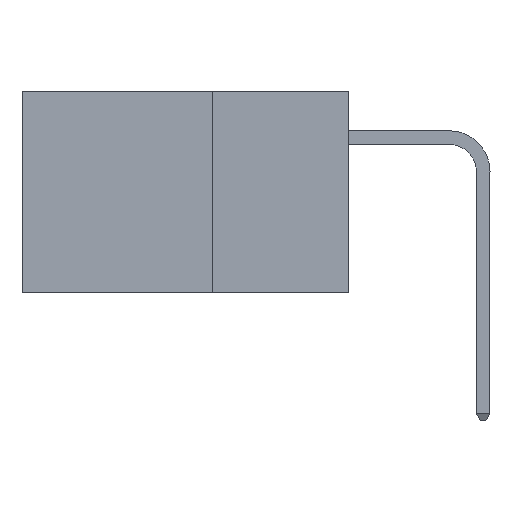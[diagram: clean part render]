
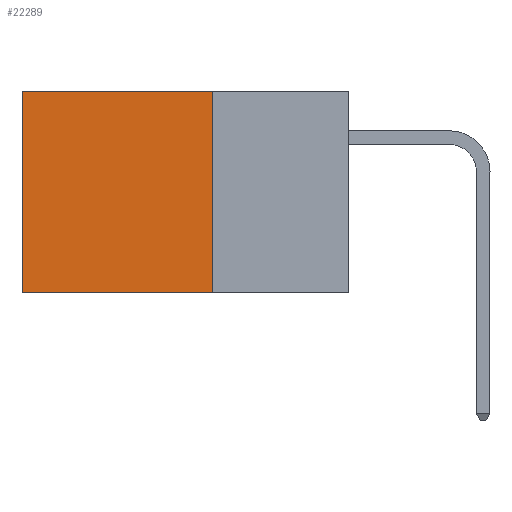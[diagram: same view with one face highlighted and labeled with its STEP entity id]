
A CAD part, left-side view. The second image highlights one B-rep face of the part: STEP entity #22289.
In plain terms, the highlighted planar face has unit normal (-1, 0, 0).
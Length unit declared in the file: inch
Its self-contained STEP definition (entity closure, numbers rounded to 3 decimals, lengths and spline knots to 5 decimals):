
#1693 = ORIENTED_EDGE ( 'NONE', *, *, #2872, .T. ) ;
#2872 = EDGE_CURVE ( 'NONE', #6135, #3264, #35801, .T. ) ;
#3264 = VERTEX_POINT ( 'NONE', #6085 ) ;
#6085 = CARTESIAN_POINT ( 'NONE',  ( 0.2875, 0.6, -0.37 ) ) ;
#6135 = VERTEX_POINT ( 'NONE', #34366 ) ;
#6524 = CARTESIAN_POINT ( 'NONE',  ( 0.2875, 0.25, -0.37 ) ) ;
#7345 = EDGE_CURVE ( 'NONE', #34507, #6135, #17134, .T. ) ;
#7349 = EDGE_CURVE ( 'NONE', #34507, #25520, #25265, .T. ) ;
#9514 = VECTOR ( 'NONE', #26277, 39.37008 ) ;
#9558 = CARTESIAN_POINT ( 'NONE',  ( 0.2875, 0.25, 0. ) ) ;
#9845 = DIRECTION ( 'NONE',  ( 1., 0., 0. ) ) ;
#12201 = VECTOR ( 'NONE', #18592, 39.37008 ) ;
#14779 = EDGE_LOOP ( 'NONE', ( #1693, #34271, #35120, #15845 ) ) ;
#15296 = DIRECTION ( 'NONE',  ( 0., 1., 0. ) ) ;
#15591 = AXIS2_PLACEMENT_3D ( 'NONE', #26546, #9845, #29298 ) ;
#15845 = ORIENTED_EDGE ( 'NONE', *, *, #7345, .T. ) ;
#17134 = LINE ( 'NONE', #31594, #9514 ) ;
#18055 = CARTESIAN_POINT ( 'NONE',  ( 0.2875, 0.25, -0.37 ) ) ;
#18592 = DIRECTION ( 'NONE',  ( 0., 0., -1. ) ) ;
#19849 = CARTESIAN_POINT ( 'NONE',  ( 0.2875, 0.25, 0. ) ) ;
#20253 = EDGE_CURVE ( 'NONE', #25520, #3264, #30960, .T. ) ;
#22289 = ADVANCED_FACE ( 'NONE', ( #27917 ), #34545, .F. ) ;
#23713 = VECTOR ( 'NONE', #15296, 39.37008 ) ;
#25265 = LINE ( 'NONE', #9558, #30795 ) ;
#25520 = VERTEX_POINT ( 'NONE', #18055 ) ;
#26277 = DIRECTION ( 'NONE',  ( 0., 1., 0. ) ) ;
#26546 = CARTESIAN_POINT ( 'NONE',  ( 0.2875, 0.25, 0. ) ) ;
#26702 = CARTESIAN_POINT ( 'NONE',  ( 0.2875, 0.6, 0. ) ) ;
#27917 = FACE_OUTER_BOUND ( 'NONE', #14779, .T. ) ;
#29298 = DIRECTION ( 'NONE',  ( 0., 0., -1. ) ) ;
#30795 = VECTOR ( 'NONE', #31696, 39.37008 ) ;
#30960 = LINE ( 'NONE', #6524, #23713 ) ;
#31594 = CARTESIAN_POINT ( 'NONE',  ( 0.2875, 0.25, 0. ) ) ;
#31696 = DIRECTION ( 'NONE',  ( 0., 0., -1. ) ) ;
#34271 = ORIENTED_EDGE ( 'NONE', *, *, #20253, .F. ) ;
#34366 = CARTESIAN_POINT ( 'NONE',  ( 0.2875, 0.6, 0. ) ) ;
#34507 = VERTEX_POINT ( 'NONE', #19849 ) ;
#34545 = PLANE ( 'NONE',  #15591 ) ;
#35120 = ORIENTED_EDGE ( 'NONE', *, *, #7349, .F. ) ;
#35801 = LINE ( 'NONE', #26702, #12201 ) ;
